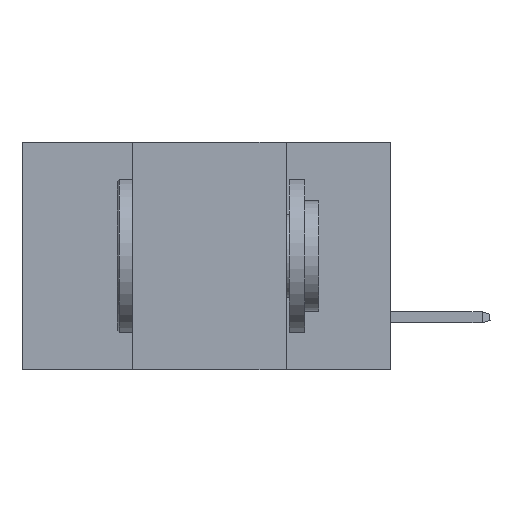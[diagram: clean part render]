
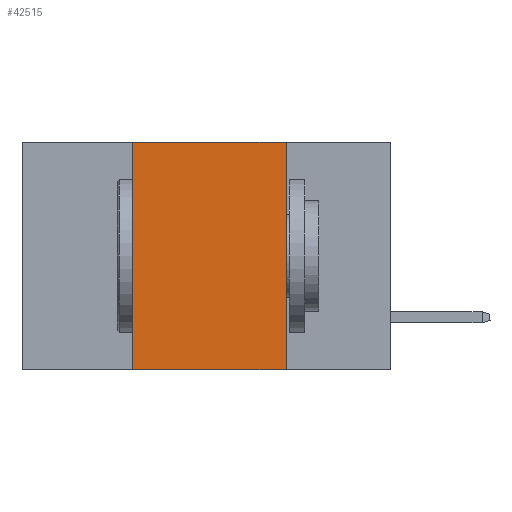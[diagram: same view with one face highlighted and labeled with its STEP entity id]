
A CAD part, left-side view. The second image highlights one B-rep face of the part: STEP entity #42515.
In plain terms, the highlighted planar face has unit normal (-1, 0, 0).
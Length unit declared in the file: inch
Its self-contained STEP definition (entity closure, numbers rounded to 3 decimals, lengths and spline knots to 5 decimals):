
#875 = PLANE ( 'NONE',  #34435 ) ;
#2614 = CARTESIAN_POINT ( 'NONE',  ( 0., 0.17, 0. ) ) ;
#2621 = VERTEX_POINT ( 'NONE', #22433 ) ;
#3962 = CARTESIAN_POINT ( 'NONE',  ( 0., 0.17, -0.37 ) ) ;
#9008 = CARTESIAN_POINT ( 'NONE',  ( 0., 0.6, -0.37 ) ) ;
#10371 = CARTESIAN_POINT ( 'NONE',  ( 0., 0.42, 0. ) ) ;
#11458 = ORIENTED_EDGE ( 'NONE', *, *, #25721, .F. ) ;
#11626 = LINE ( 'NONE', #9008, #32710 ) ;
#12685 = DIRECTION ( 'NONE',  ( 0., -1., 0. ) ) ;
#15335 = FACE_OUTER_BOUND ( 'NONE', #38156, .T. ) ;
#15554 = DIRECTION ( 'NONE',  ( 0., 0., -1. ) ) ;
#16717 = DIRECTION ( 'NONE',  ( 0., -1., 0. ) ) ;
#17705 = DIRECTION ( 'NONE',  ( 0., 0., 1. ) ) ;
#19145 = VECTOR ( 'NONE', #17705, 39.37008 ) ;
#20418 = ORIENTED_EDGE ( 'NONE', *, *, #36263, .T. ) ;
#22433 = CARTESIAN_POINT ( 'NONE',  ( 0., 0.17, 0. ) ) ;
#25618 = ORIENTED_EDGE ( 'NONE', *, *, #29652, .F. ) ;
#25662 = CARTESIAN_POINT ( 'NONE',  ( 0., 0.42, 0. ) ) ;
#25721 = EDGE_CURVE ( 'NONE', #2621, #32503, #30355, .T. ) ;
#28196 = EDGE_CURVE ( 'NONE', #44740, #2621, #44354, .T. ) ;
#28635 = CARTESIAN_POINT ( 'NONE',  ( 0., 0.42, -0.37 ) ) ;
#28651 = ORIENTED_EDGE ( 'NONE', *, *, #28196, .F. ) ;
#29558 = CARTESIAN_POINT ( 'NONE',  ( 0., 0.6, 0. ) ) ;
#29652 = EDGE_CURVE ( 'NONE', #38236, #44740, #47190, .T. ) ;
#30355 = LINE ( 'NONE', #2614, #42922 ) ;
#30690 = VECTOR ( 'NONE', #16717, 39.37008 ) ;
#32503 = VERTEX_POINT ( 'NONE', #3962 ) ;
#32710 = VECTOR ( 'NONE', #12685, 39.37008 ) ;
#34435 = AXIS2_PLACEMENT_3D ( 'NONE', #29558, #44413, #15554 ) ;
#35127 = DIRECTION ( 'NONE',  ( 0., 0., -1. ) ) ;
#36263 = EDGE_CURVE ( 'NONE', #38236, #32503, #11626, .T. ) ;
#38156 = EDGE_LOOP ( 'NONE', ( #11458, #28651, #25618, #20418 ) ) ;
#38236 = VERTEX_POINT ( 'NONE', #28635 ) ;
#42515 = ADVANCED_FACE ( 'NONE', ( #15335 ), #875, .F. ) ;
#42922 = VECTOR ( 'NONE', #35127, 39.37008 ) ;
#44354 = LINE ( 'NONE', #46269, #30690 ) ;
#44413 = DIRECTION ( 'NONE',  ( 1., 0., 0. ) ) ;
#44740 = VERTEX_POINT ( 'NONE', #25662 ) ;
#46269 = CARTESIAN_POINT ( 'NONE',  ( 0., 0.6, 0. ) ) ;
#47190 = LINE ( 'NONE', #10371, #19145 ) ;
